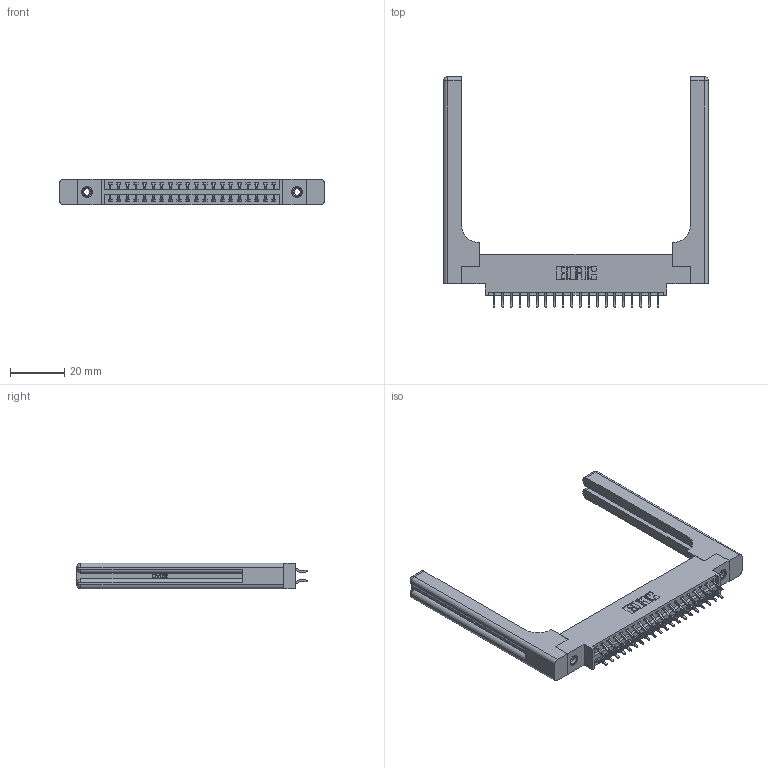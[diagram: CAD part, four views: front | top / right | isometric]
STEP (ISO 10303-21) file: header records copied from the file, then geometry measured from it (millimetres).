
FILE_DESCRIPTION (( 'STEP AP203' ), '1' );
FILE_NAME ('346-040-556-858.STEP', '2022-05-20T02:43:12', ( '' ), ( '' ), 'SwSTEP 2.0', 'SolidWorks 2020', '' );
FILE_SCHEMA (( 'CONFIG_CONTROL_DESIGN' ));
Length unit declared in the file: inch
Products named in the file (5): 346-220-058_345-220-058; 346 Part_0.170 Offset - 0.156 Dia-TH; 346-040-556-858; 345-250-001_345-250-001-102; 345-292-001_556 Tail
Assembly tree (45 placements, depth 2):
  346-040-556-858
    346 Part_0.170 Offset - 0.156 Dia-TH
    345-292-001_556 Tail  x40
    345-250-001_345-250-001-102  x2
    346-220-058_345-220-058  x2
Bounding box: 97.56 x 84.84 x 9.4 mm (x, y, z)
Volume: 16662.5 mm3; surface area: 17406.4 mm2
Topology: 45 solids, 45 shells, 2716 faces, 7963 edges, 5234 vertices
Faces by surface type: plane 1802, cylinder 854, bspline 36, cone 12, sphere 8, torus 4
Entity records: 21964 total; most frequent: CARTESIAN_POINT 4679, ORIENTED_EDGE 3396, DIRECTION 3094, EDGE_CURVE 1698, LINE 1386, VECTOR 1386, VERTEX_POINT 1122, AXIS2_PLACEMENT_3D 854
